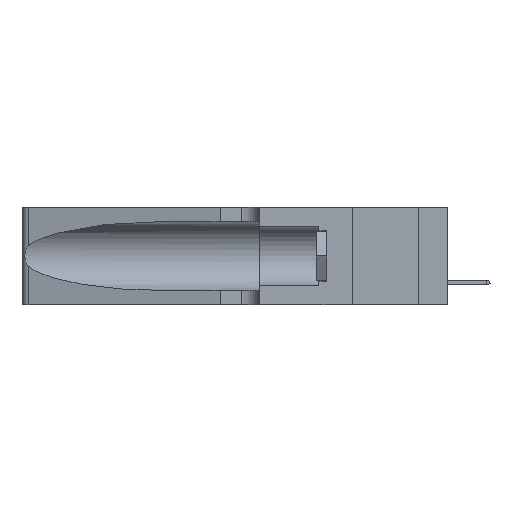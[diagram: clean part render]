
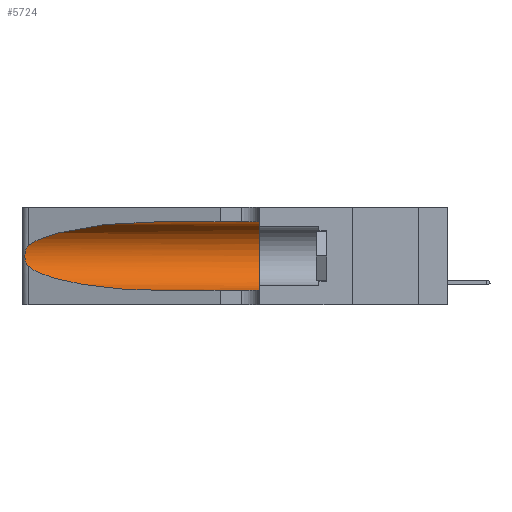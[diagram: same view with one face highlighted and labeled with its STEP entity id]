
A CAD part, left-side view. The second image highlights one B-rep face of the part: STEP entity #5724.
In plain terms, the highlighted cylindrical face has radius 3.308 mm (diameter 6.617 mm), a partial arc.
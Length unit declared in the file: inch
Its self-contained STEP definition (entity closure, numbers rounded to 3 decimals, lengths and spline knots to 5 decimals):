
#1035 = CARTESIAN_POINT ( 'NONE',  ( 0.1305, 0.35, 0.31525 ) ) ;
#2573 =( BOUNDED_CURVE ( )  B_SPLINE_CURVE ( 3, ( #38273, #22161, #22343, #14548 ),
 .UNSPECIFIED., .F., .F. ) 
 B_SPLINE_CURVE_WITH_KNOTS ( ( 4, 4 ),
 ( 1.5708, 2.84003 ),
 .UNSPECIFIED. ) 
 CURVE ( )  GEOMETRIC_REPRESENTATION_ITEM ( )  RATIONAL_B_SPLINE_CURVE ( ( 1., 0.87, 0.87, 1. ) ) 
 REPRESENTATION_ITEM ( '' )  );
#2594 = CARTESIAN_POINT ( 'NONE',  ( 0.25487, 1.22718, 0.14631 ) ) ;
#2904 = ORIENTED_EDGE ( 'NONE', *, *, #28232, .F. ) ;
#3278 = B_SPLINE_CURVE_WITH_KNOTS ( 'NONE', 3,
 ( #34349, #26498, #38477, #17975, #39591, #28914, #21487, #3534, #40475, #37723, #19400, #47048, #28148, #4710 ),
 .UNSPECIFIED., .F., .F.,
 ( 4, 2, 2, 2, 2, 2, 4 ),
 ( 0., 0.00027, 0.00053, 0.00107, 0.0016, 0.00187, 0.00214 ),
 .UNSPECIFIED. ) ;
#3534 = CARTESIAN_POINT ( 'NONE',  ( 0.26075, 1.23896, 0.178 ) ) ;
#3552 = AXIS2_PLACEMENT_3D ( 'NONE', #7994, #35555, #39677 ) ;
#4710 = CARTESIAN_POINT ( 'NONE',  ( 0.25487, 1.22718, 0.14631 ) ) ;
#5096 = EDGE_CURVE ( 'NONE', #5417, #22662, #27793, .T. ) ;
#5417 = VERTEX_POINT ( 'NONE', #31285 ) ;
#5724 = ADVANCED_FACE ( 'NONE', ( #50052 ), #46298, .F. ) ;
#6431 = CARTESIAN_POINT ( 'NONE',  ( 0.2373, 1.15595, 0.08982 ) ) ;
#7579 = ORIENTED_EDGE ( 'NONE', *, *, #5096, .F. ) ;
#7994 = CARTESIAN_POINT ( 'NONE',  ( 0.1305, 1.61858, 0.185 ) ) ;
#8811 = EDGE_LOOP ( 'NONE', ( #36960, #16162, #38592, #22817, #2904, #7579 ) ) ;
#14548 = CARTESIAN_POINT ( 'NONE',  ( 0.25487, 1.22718, 0.22369 ) ) ;
#14933 = CARTESIAN_POINT ( 'NONE',  ( 0.1305, 0.72297, 0.05475 ) ) ;
#15111 = CARTESIAN_POINT ( 'NONE',  ( 0.1305, 1.61858, 0.31525 ) ) ;
#16162 = ORIENTED_EDGE ( 'NONE', *, *, #28720, .T. ) ;
#17371 = CARTESIAN_POINT ( 'NONE',  ( 0.25487, 1.22718, 0.14631 ) ) ;
#17975 = CARTESIAN_POINT ( 'NONE',  ( 0.25787, 1.23484, 0.2124 ) ) ;
#18783 = VECTOR ( 'NONE', #42289, 39.37008 ) ;
#19400 = CARTESIAN_POINT ( 'NONE',  ( 0.25789, 1.23486, 0.15765 ) ) ;
#19969 = EDGE_CURVE ( 'NONE', #40199, #40113, #29216, .T. ) ;
#21487 = CARTESIAN_POINT ( 'NONE',  ( 0.26075, 1.23896, 0.19203 ) ) ;
#22161 = CARTESIAN_POINT ( 'NONE',  ( 0.18966, 0.96281, 0.31525 ) ) ;
#22343 = CARTESIAN_POINT ( 'NONE',  ( 0.2373, 1.15595, 0.28018 ) ) ;
#22662 = VERTEX_POINT ( 'NONE', #1035 ) ;
#22817 = ORIENTED_EDGE ( 'NONE', *, *, #19969, .T. ) ;
#22868 = CARTESIAN_POINT ( 'NONE',  ( 0.1305, 0.72297, 0.05475 ) ) ;
#26439 = CARTESIAN_POINT ( 'NONE',  ( 0.25487, 1.22718, 0.22369 ) ) ;
#26498 = CARTESIAN_POINT ( 'NONE',  ( 0.25555, 1.22994, 0.2215 ) ) ;
#26634 = DIRECTION ( 'NONE',  ( 0., 0., 1. ) ) ;
#27793 = LINE ( 'NONE', #15111, #42038 ) ;
#28148 = CARTESIAN_POINT ( 'NONE',  ( 0.25555, 1.22993, 0.14849 ) ) ;
#28232 = EDGE_CURVE ( 'NONE', #22662, #40113, #28513, .T. ) ;
#28513 = CIRCLE ( 'NONE', #49921, 0.13025 ) ;
#28720 = EDGE_CURVE ( 'NONE', #50285, #37699, #3278, .T. ) ;
#28914 = CARTESIAN_POINT ( 'NONE',  ( 0.26018, 1.23835, 0.19895 ) ) ;
#29216 = LINE ( 'NONE', #30176, #18783 ) ;
#30176 = CARTESIAN_POINT ( 'NONE',  ( 0.1305, 1.61858, 0.05475 ) ) ;
#31285 = CARTESIAN_POINT ( 'NONE',  ( 0.1305, 0.72297, 0.31525 ) ) ;
#34210 = DIRECTION ( 'NONE',  ( 0., -1., 0. ) ) ;
#34349 = CARTESIAN_POINT ( 'NONE',  ( 0.25487, 1.22718, 0.22369 ) ) ;
#34530 = CARTESIAN_POINT ( 'NONE',  ( 0.18966, 0.96281, 0.05475 ) ) ;
#35555 = DIRECTION ( 'NONE',  ( 0., -1., 0. ) ) ;
#36960 = ORIENTED_EDGE ( 'NONE', *, *, #49761, .T. ) ;
#37090 = EDGE_CURVE ( 'NONE', #37699, #40199, #45357, .T. ) ;
#37699 = VERTEX_POINT ( 'NONE', #17371 ) ;
#37723 = CARTESIAN_POINT ( 'NONE',  ( 0.25856, 1.23593, 0.16098 ) ) ;
#38273 = CARTESIAN_POINT ( 'NONE',  ( 0.1305, 0.72297, 0.31525 ) ) ;
#38477 = CARTESIAN_POINT ( 'NONE',  ( 0.25639, 1.23184, 0.21858 ) ) ;
#38592 = ORIENTED_EDGE ( 'NONE', *, *, #37090, .T. ) ;
#39591 = CARTESIAN_POINT ( 'NONE',  ( 0.25854, 1.2359, 0.20912 ) ) ;
#39677 = DIRECTION ( 'NONE',  ( 0., 0., -1. ) ) ;
#39928 = CARTESIAN_POINT ( 'NONE',  ( 0.1305, 0.35, 0.185 ) ) ;
#40113 = VERTEX_POINT ( 'NONE', #46003 ) ;
#40199 = VERTEX_POINT ( 'NONE', #22868 ) ;
#40475 = CARTESIAN_POINT ( 'NONE',  ( 0.26017, 1.23833, 0.17102 ) ) ;
#42038 = VECTOR ( 'NONE', #34210, 39.37008 ) ;
#42289 = DIRECTION ( 'NONE',  ( 0., -1., 0. ) ) ;
#45357 =( BOUNDED_CURVE ( )  B_SPLINE_CURVE ( 3, ( #2594, #6431, #34530, #14933 ),
 .UNSPECIFIED., .F., .T. ) 
 B_SPLINE_CURVE_WITH_KNOTS ( ( 4, 4 ),
 ( 3.44316, 4.71239 ),
 .UNSPECIFIED. ) 
 CURVE ( )  GEOMETRIC_REPRESENTATION_ITEM ( )  RATIONAL_B_SPLINE_CURVE ( ( 1., 0.87, 0.87, 1. ) ) 
 REPRESENTATION_ITEM ( '' )  );
#46003 = CARTESIAN_POINT ( 'NONE',  ( 0.1305, 0.35, 0.05475 ) ) ;
#46298 = CYLINDRICAL_SURFACE ( 'NONE', #3552, 0.13025 ) ;
#46304 = DIRECTION ( 'NONE',  ( 0., 1., 0. ) ) ;
#47048 = CARTESIAN_POINT ( 'NONE',  ( 0.25639, 1.23186, 0.15144 ) ) ;
#49761 = EDGE_CURVE ( 'NONE', #5417, #50285, #2573, .T. ) ;
#49921 = AXIS2_PLACEMENT_3D ( 'NONE', #39928, #46304, #26634 ) ;
#50052 = FACE_OUTER_BOUND ( 'NONE', #8811, .T. ) ;
#50285 = VERTEX_POINT ( 'NONE', #26439 ) ;
